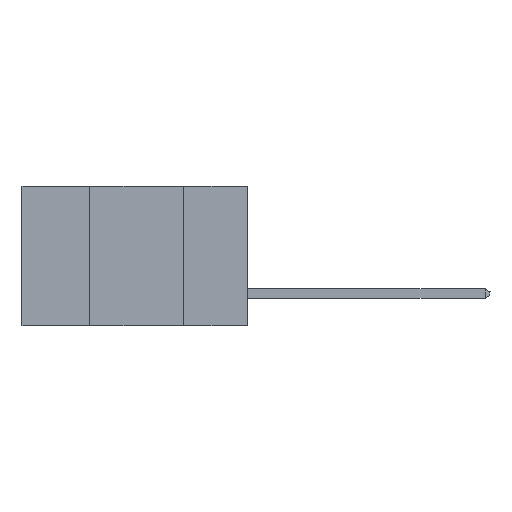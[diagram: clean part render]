
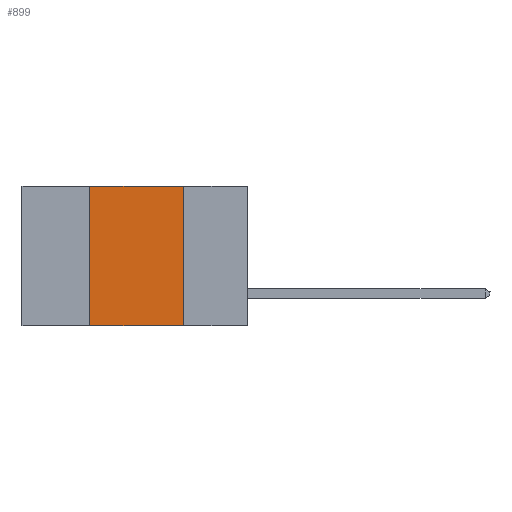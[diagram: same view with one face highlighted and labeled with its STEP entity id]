
A CAD part, left-side view. The second image highlights one B-rep face of the part: STEP entity #899.
In plain terms, the highlighted planar face has unit normal (-1, 0, 0).
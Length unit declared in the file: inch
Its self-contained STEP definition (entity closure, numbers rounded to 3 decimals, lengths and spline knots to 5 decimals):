
#721 = DIRECTION ( 'NONE',  ( 0., 0., -1. ) ) ;
#726 = CARTESIAN_POINT ( 'NONE',  ( 0., 0.6, 0. ) ) ;
#899 = ADVANCED_FACE ( 'NONE', ( #11013 ), #13852, .F. ) ;
#1065 = EDGE_CURVE ( 'NONE', #5024, #13623, #15312, .T. ) ;
#1364 = VECTOR ( 'NONE', #15678, 39.37008 ) ;
#1529 = LINE ( 'NONE', #8083, #20174 ) ;
#3232 = CARTESIAN_POINT ( 'NONE',  ( 0., 0.17, 0. ) ) ;
#3963 = CARTESIAN_POINT ( 'NONE',  ( 0., 0.42, 0. ) ) ;
#4000 = CARTESIAN_POINT ( 'NONE',  ( 0., 0.6, -0.37 ) ) ;
#4818 = EDGE_CURVE ( 'NONE', #12110, #13623, #13077, .T. ) ;
#5024 = VERTEX_POINT ( 'NONE', #19730 ) ;
#5569 = DIRECTION ( 'NONE',  ( 1., 0., 0. ) ) ;
#5618 = ORIENTED_EDGE ( 'NONE', *, *, #17135, .F. ) ;
#5778 = ORIENTED_EDGE ( 'NONE', *, *, #4818, .F. ) ;
#8083 = CARTESIAN_POINT ( 'NONE',  ( 0., 0.42, -0.37 ) ) ;
#8285 = DIRECTION ( 'NONE',  ( 0., 0., 1. ) ) ;
#10021 = EDGE_LOOP ( 'NONE', ( #5778, #5618, #10327, #19566 ) ) ;
#10327 = ORIENTED_EDGE ( 'NONE', *, *, #15219, .F. ) ;
#11013 = FACE_OUTER_BOUND ( 'NONE', #10021, .T. ) ;
#11378 = AXIS2_PLACEMENT_3D ( 'NONE', #15969, #5569, #721 ) ;
#12110 = VERTEX_POINT ( 'NONE', #3232 ) ;
#13077 = LINE ( 'NONE', #21140, #16662 ) ;
#13623 = VERTEX_POINT ( 'NONE', #16581 ) ;
#13852 = PLANE ( 'NONE',  #11378 ) ;
#15154 = VECTOR ( 'NONE', #18624, 39.37008 ) ;
#15219 = EDGE_CURVE ( 'NONE', #5024, #18926, #1529, .T. ) ;
#15312 = LINE ( 'NONE', #4000, #15154 ) ;
#15678 = DIRECTION ( 'NONE',  ( 0., -1., 0. ) ) ;
#15969 = CARTESIAN_POINT ( 'NONE',  ( 0., 0.6, 0. ) ) ;
#16581 = CARTESIAN_POINT ( 'NONE',  ( 0., 0.17, -0.37 ) ) ;
#16662 = VECTOR ( 'NONE', #21039, 39.37008 ) ;
#17135 = EDGE_CURVE ( 'NONE', #18926, #12110, #18460, .T. ) ;
#18460 = LINE ( 'NONE', #726, #1364 ) ;
#18624 = DIRECTION ( 'NONE',  ( 0., -1., 0. ) ) ;
#18926 = VERTEX_POINT ( 'NONE', #3963 ) ;
#19566 = ORIENTED_EDGE ( 'NONE', *, *, #1065, .T. ) ;
#19730 = CARTESIAN_POINT ( 'NONE',  ( 0., 0.42, -0.37 ) ) ;
#20174 = VECTOR ( 'NONE', #8285, 39.37008 ) ;
#21039 = DIRECTION ( 'NONE',  ( 0., 0., -1. ) ) ;
#21140 = CARTESIAN_POINT ( 'NONE',  ( 0., 0.17, -0.37 ) ) ;
